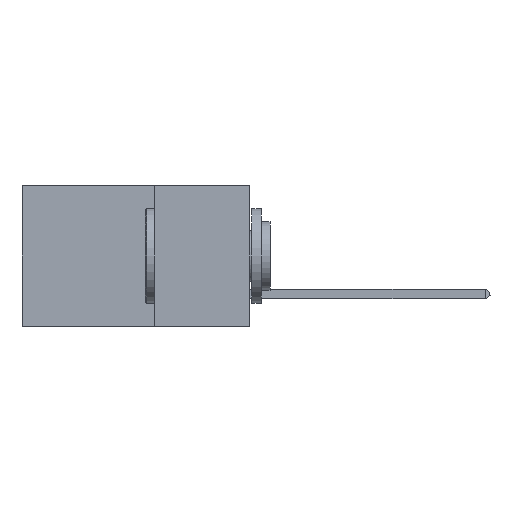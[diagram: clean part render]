
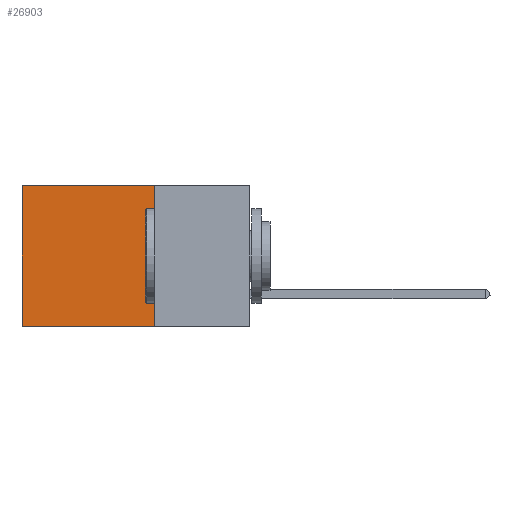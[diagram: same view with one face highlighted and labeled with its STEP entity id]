
A CAD part, left-side view. The second image highlights one B-rep face of the part: STEP entity #26903.
In plain terms, the highlighted planar face has unit normal (-1, 0, 0).
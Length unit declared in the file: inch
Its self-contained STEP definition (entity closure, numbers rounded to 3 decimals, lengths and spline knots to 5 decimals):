
#709 = CARTESIAN_POINT ( 'NONE',  ( 0.2875, 0.6, 0. ) ) ;
#2470 = EDGE_CURVE ( 'NONE', #24524, #7575, #30221, .T. ) ;
#2555 = CARTESIAN_POINT ( 'NONE',  ( 0.2875, 0.6, -0.37 ) ) ;
#5839 = CARTESIAN_POINT ( 'NONE',  ( 0.2875, 0.6, 0. ) ) ;
#5991 = FACE_OUTER_BOUND ( 'NONE', #24383, .T. ) ;
#7575 = VERTEX_POINT ( 'NONE', #5839 ) ;
#8342 = DIRECTION ( 'NONE',  ( 1., 0., 0. ) ) ;
#9724 = CARTESIAN_POINT ( 'NONE',  ( 0.2875, 0.25, 0. ) ) ;
#10954 = PLANE ( 'NONE',  #20030 ) ;
#11060 = DIRECTION ( 'NONE',  ( 0., 0., -1. ) ) ;
#11586 = VERTEX_POINT ( 'NONE', #18252 ) ;
#11619 = ORIENTED_EDGE ( 'NONE', *, *, #14304, .T. ) ;
#12728 = VECTOR ( 'NONE', #14992, 39.37008 ) ;
#12806 = EDGE_CURVE ( 'NONE', #24524, #11586, #14355, .T. ) ;
#13007 = LINE ( 'NONE', #28040, #32831 ) ;
#13250 = DIRECTION ( 'NONE',  ( 0., 0., -1. ) ) ;
#13838 = VECTOR ( 'NONE', #13250, 39.37008 ) ;
#13895 = CARTESIAN_POINT ( 'NONE',  ( 0.2875, 0.25, 0. ) ) ;
#14304 = EDGE_CURVE ( 'NONE', #7575, #32035, #31207, .T. ) ;
#14355 = LINE ( 'NONE', #30449, #12728 ) ;
#14992 = DIRECTION ( 'NONE',  ( 0., 0., -1. ) ) ;
#17794 = EDGE_CURVE ( 'NONE', #11586, #32035, #13007, .T. ) ;
#18252 = CARTESIAN_POINT ( 'NONE',  ( 0.2875, 0.25, -0.37 ) ) ;
#20030 = AXIS2_PLACEMENT_3D ( 'NONE', #13895, #8342, #11060 ) ;
#21137 = DIRECTION ( 'NONE',  ( 0., 1., 0. ) ) ;
#22947 = VECTOR ( 'NONE', #28221, 39.37008 ) ;
#23853 = ORIENTED_EDGE ( 'NONE', *, *, #2470, .T. ) ;
#24383 = EDGE_LOOP ( 'NONE', ( #11619, #31621, #29066, #23853 ) ) ;
#24524 = VERTEX_POINT ( 'NONE', #9724 ) ;
#25635 = CARTESIAN_POINT ( 'NONE',  ( 0.2875, 0.25, 0. ) ) ;
#26903 = ADVANCED_FACE ( 'NONE', ( #5991 ), #10954, .F. ) ;
#28040 = CARTESIAN_POINT ( 'NONE',  ( 0.2875, 0.25, -0.37 ) ) ;
#28221 = DIRECTION ( 'NONE',  ( 0., 1., 0. ) ) ;
#29066 = ORIENTED_EDGE ( 'NONE', *, *, #12806, .F. ) ;
#30221 = LINE ( 'NONE', #25635, #22947 ) ;
#30449 = CARTESIAN_POINT ( 'NONE',  ( 0.2875, 0.25, 0. ) ) ;
#31207 = LINE ( 'NONE', #709, #13838 ) ;
#31621 = ORIENTED_EDGE ( 'NONE', *, *, #17794, .F. ) ;
#32035 = VERTEX_POINT ( 'NONE', #2555 ) ;
#32831 = VECTOR ( 'NONE', #21137, 39.37008 ) ;
